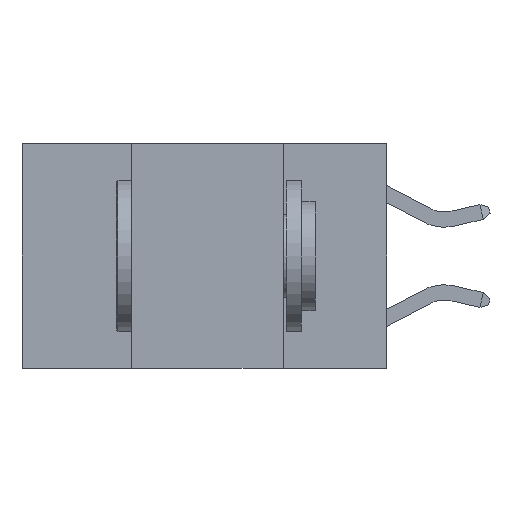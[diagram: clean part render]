
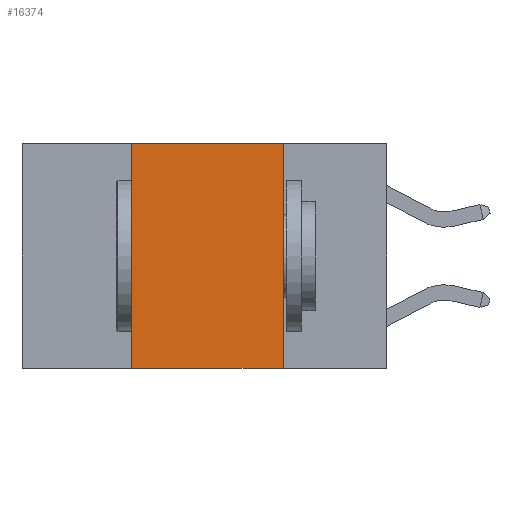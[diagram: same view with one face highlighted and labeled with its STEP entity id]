
A CAD part, left-side view. The second image highlights one B-rep face of the part: STEP entity #16374.
In plain terms, the highlighted planar face has unit normal (-1, 0, 0).
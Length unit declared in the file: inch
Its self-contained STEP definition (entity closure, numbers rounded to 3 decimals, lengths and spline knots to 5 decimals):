
#2163 = DIRECTION ( 'NONE',  ( 1., 0., 0. ) ) ;
#2992 = CARTESIAN_POINT ( 'NONE',  ( 0., 0.17, -0.37 ) ) ;
#3401 = AXIS2_PLACEMENT_3D ( 'NONE', #15117, #2163, #17254 ) ;
#3736 = EDGE_CURVE ( 'NONE', #12323, #4776, #16810, .T. ) ;
#4393 = FACE_OUTER_BOUND ( 'NONE', #17655, .T. ) ;
#4776 = VERTEX_POINT ( 'NONE', #2992 ) ;
#7419 = CARTESIAN_POINT ( 'NONE',  ( 0., 0.42, 0. ) ) ;
#8324 = DIRECTION ( 'NONE',  ( 0., 0., 1. ) ) ;
#9088 = CARTESIAN_POINT ( 'NONE',  ( 0., 0.17, 0. ) ) ;
#9223 = VECTOR ( 'NONE', #8324, 39.37008 ) ;
#10297 = ORIENTED_EDGE ( 'NONE', *, *, #3736, .F. ) ;
#10488 = VECTOR ( 'NONE', #22971, 39.37008 ) ;
#10880 = DIRECTION ( 'NONE',  ( 0., -1., 0. ) ) ;
#11691 = EDGE_CURVE ( 'NONE', #13865, #12323, #25639, .T. ) ;
#11993 = LINE ( 'NONE', #25810, #16309 ) ;
#12323 = VERTEX_POINT ( 'NONE', #9088 ) ;
#13865 = VERTEX_POINT ( 'NONE', #7419 ) ;
#14282 = EDGE_CURVE ( 'NONE', #19574, #4776, #11993, .T. ) ;
#15117 = CARTESIAN_POINT ( 'NONE',  ( 0., 0.6, 0. ) ) ;
#15703 = EDGE_CURVE ( 'NONE', #19574, #13865, #26261, .T. ) ;
#16309 = VECTOR ( 'NONE', #10880, 39.37008 ) ;
#16374 = ADVANCED_FACE ( 'NONE', ( #4393 ), #17171, .F. ) ;
#16529 = CARTESIAN_POINT ( 'NONE',  ( 0., 0.17, 0. ) ) ;
#16810 = LINE ( 'NONE', #16529, #10488 ) ;
#17171 = PLANE ( 'NONE',  #3401 ) ;
#17254 = DIRECTION ( 'NONE',  ( 0., 0., -1. ) ) ;
#17291 = ORIENTED_EDGE ( 'NONE', *, *, #15703, .F. ) ;
#17655 = EDGE_LOOP ( 'NONE', ( #10297, #22296, #17291, #23641 ) ) ;
#19574 = VERTEX_POINT ( 'NONE', #23981 ) ;
#19652 = DIRECTION ( 'NONE',  ( 0., -1., 0. ) ) ;
#21809 = CARTESIAN_POINT ( 'NONE',  ( 0., 0.6, 0. ) ) ;
#22296 = ORIENTED_EDGE ( 'NONE', *, *, #11691, .F. ) ;
#22971 = DIRECTION ( 'NONE',  ( 0., 0., -1. ) ) ;
#23351 = CARTESIAN_POINT ( 'NONE',  ( 0., 0.42, 0. ) ) ;
#23641 = ORIENTED_EDGE ( 'NONE', *, *, #14282, .T. ) ;
#23981 = CARTESIAN_POINT ( 'NONE',  ( 0., 0.42, -0.37 ) ) ;
#25639 = LINE ( 'NONE', #21809, #26312 ) ;
#25810 = CARTESIAN_POINT ( 'NONE',  ( 0., 0.6, -0.37 ) ) ;
#26261 = LINE ( 'NONE', #23351, #9223 ) ;
#26312 = VECTOR ( 'NONE', #19652, 39.37008 ) ;
